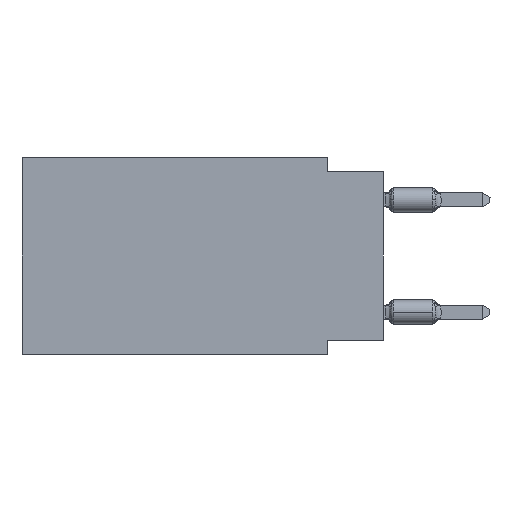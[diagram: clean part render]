
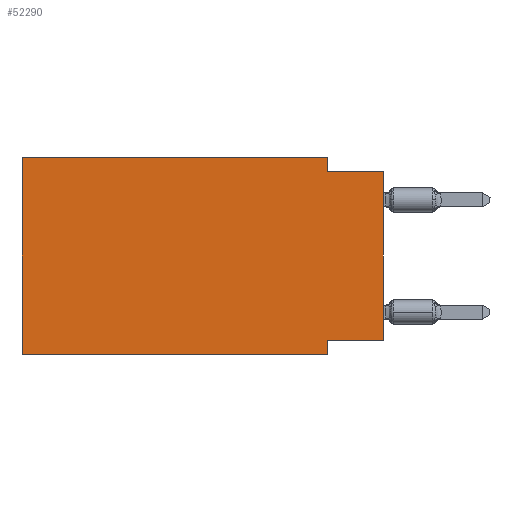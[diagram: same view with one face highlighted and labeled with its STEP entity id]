
A CAD part, left-side view. The second image highlights one B-rep face of the part: STEP entity #52290.
In plain terms, the highlighted planar face has unit normal (-1, 0, 0).
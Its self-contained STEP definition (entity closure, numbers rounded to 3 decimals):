
#23 = VERTEX_POINT ( 'NONE', #41045 ) ;
#715 = EDGE_CURVE ( 'NONE', #12150, #25391, #11235, .T. ) ;
#2665 = DIRECTION ( 'NONE',  ( 0., 0., -1. ) ) ;
#6123 = ORIENTED_EDGE ( 'NONE', *, *, #26719, .F. ) ;
#6523 = DIRECTION ( 'NONE',  ( 0., -1., 0. ) ) ;
#8339 = VECTOR ( 'NONE', #45317, 1000. ) ;
#8928 = DIRECTION ( 'NONE',  ( 0., -1., 0. ) ) ;
#11077 = LINE ( 'NONE', #48027, #47119 ) ;
#11235 = LINE ( 'NONE', #29708, #30050 ) ;
#12150 = VERTEX_POINT ( 'NONE', #25306 ) ;
#14087 = VERTEX_POINT ( 'NONE', #35832 ) ;
#15025 = CARTESIAN_POINT ( 'NONE',  ( 0., 2.54, 0. ) ) ;
#15366 = VERTEX_POINT ( 'NONE', #23061 ) ;
#17255 = DIRECTION ( 'NONE',  ( 0., 1., 0. ) ) ;
#17669 = VERTEX_POINT ( 'NONE', #15025 ) ;
#17798 = CARTESIAN_POINT ( 'NONE',  ( 0., 2.54, 0. ) ) ;
#18322 = CARTESIAN_POINT ( 'NONE',  ( 0., 16.383, -8.89 ) ) ;
#19538 = LINE ( 'NONE', #24661, #39285 ) ;
#20491 = CARTESIAN_POINT ( 'NONE',  ( 0., 2.54, -8.89 ) ) ;
#21475 = EDGE_LOOP ( 'NONE', ( #47342, #43513, #28500, #27340, #35328, #27176, #45408, #6123 ) ) ;
#22702 = PLANE ( 'NONE',  #58815 ) ;
#22717 = DIRECTION ( 'NONE',  ( 0., 0., 1. ) ) ;
#22848 = EDGE_CURVE ( 'NONE', #12150, #35604, #31637, .T. ) ;
#23061 = CARTESIAN_POINT ( 'NONE',  ( 0., 0., -8.255 ) ) ;
#23140 = DIRECTION ( 'NONE',  ( 0., 0., 1. ) ) ;
#23233 = CARTESIAN_POINT ( 'NONE',  ( 0., 2.54, -8.255 ) ) ;
#24661 = CARTESIAN_POINT ( 'NONE',  ( 0., 0., -0.635 ) ) ;
#25306 = CARTESIAN_POINT ( 'NONE',  ( 0., 16.383, -8.89 ) ) ;
#25391 = VERTEX_POINT ( 'NONE', #29092 ) ;
#26719 = EDGE_CURVE ( 'NONE', #15366, #52700, #31184, .T. ) ;
#27176 = ORIENTED_EDGE ( 'NONE', *, *, #22848, .T. ) ;
#27340 = ORIENTED_EDGE ( 'NONE', *, *, #59280, .F. ) ;
#27985 = LINE ( 'NONE', #42522, #52622 ) ;
#28231 = VECTOR ( 'NONE', #8928, 1000. ) ;
#28500 = ORIENTED_EDGE ( 'NONE', *, *, #38991, .F. ) ;
#29092 = CARTESIAN_POINT ( 'NONE',  ( 0., 16.383, 0. ) ) ;
#29708 = CARTESIAN_POINT ( 'NONE',  ( 0., 16.383, 0. ) ) ;
#30050 = VECTOR ( 'NONE', #22717, 1000. ) ;
#31184 = LINE ( 'NONE', #40264, #45371 ) ;
#31373 = CARTESIAN_POINT ( 'NONE',  ( 0., 2.54, -8.89 ) ) ;
#31637 = LINE ( 'NONE', #18322, #28231 ) ;
#35328 = ORIENTED_EDGE ( 'NONE', *, *, #715, .F. ) ;
#35604 = VERTEX_POINT ( 'NONE', #20491 ) ;
#35832 = CARTESIAN_POINT ( 'NONE',  ( 0., 2.54, -0.635 ) ) ;
#38991 = EDGE_CURVE ( 'NONE', #17669, #14087, #59312, .T. ) ;
#39285 = VECTOR ( 'NONE', #56505, 1000. ) ;
#40264 = CARTESIAN_POINT ( 'NONE',  ( 0., 0., -8.255 ) ) ;
#41045 = CARTESIAN_POINT ( 'NONE',  ( 0., 0., -0.635 ) ) ;
#42522 = CARTESIAN_POINT ( 'NONE',  ( 0., 0., 0. ) ) ;
#43513 = ORIENTED_EDGE ( 'NONE', *, *, #45903, .F. ) ;
#45317 = DIRECTION ( 'NONE',  ( 0., 0., -1. ) ) ;
#45371 = VECTOR ( 'NONE', #17255, 1000. ) ;
#45408 = ORIENTED_EDGE ( 'NONE', *, *, #45679, .F. ) ;
#45679 = EDGE_CURVE ( 'NONE', #52700, #35604, #58361, .T. ) ;
#45903 = EDGE_CURVE ( 'NONE', #14087, #23, #19538, .T. ) ;
#46930 = DIRECTION ( 'NONE',  ( 0., 0., -1. ) ) ;
#47119 = VECTOR ( 'NONE', #6523, 1000. ) ;
#47342 = ORIENTED_EDGE ( 'NONE', *, *, #54232, .T. ) ;
#48027 = CARTESIAN_POINT ( 'NONE',  ( 0., 16.383, 0. ) ) ;
#52290 = ADVANCED_FACE ( 'NONE', ( #55713 ), #22702, .F. ) ;
#52622 = VECTOR ( 'NONE', #23140, 1000. ) ;
#52700 = VERTEX_POINT ( 'NONE', #23233 ) ;
#54232 = EDGE_CURVE ( 'NONE', #15366, #23, #27985, .T. ) ;
#55423 = DIRECTION ( 'NONE',  ( 1., 0., 0. ) ) ;
#55713 = FACE_OUTER_BOUND ( 'NONE', #21475, .T. ) ;
#56505 = DIRECTION ( 'NONE',  ( 0., -1., 0. ) ) ;
#58099 = VECTOR ( 'NONE', #2665, 1000. ) ;
#58361 = LINE ( 'NONE', #31373, #8339 ) ;
#58815 = AXIS2_PLACEMENT_3D ( 'NONE', #59659, #55423, #46930 ) ;
#59280 = EDGE_CURVE ( 'NONE', #25391, #17669, #11077, .T. ) ;
#59312 = LINE ( 'NONE', #17798, #58099 ) ;
#59659 = CARTESIAN_POINT ( 'NONE',  ( 0., 16.383, 0. ) ) ;
